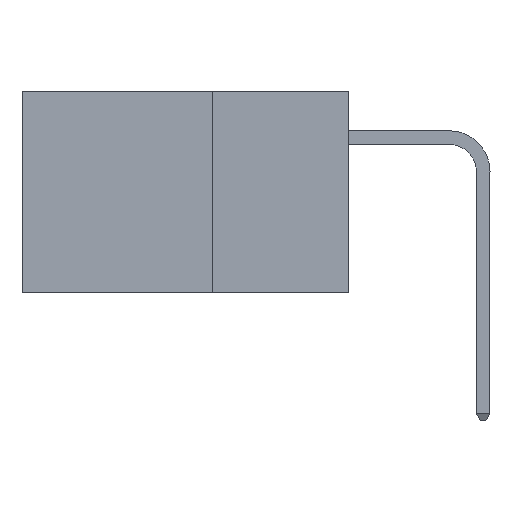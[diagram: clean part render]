
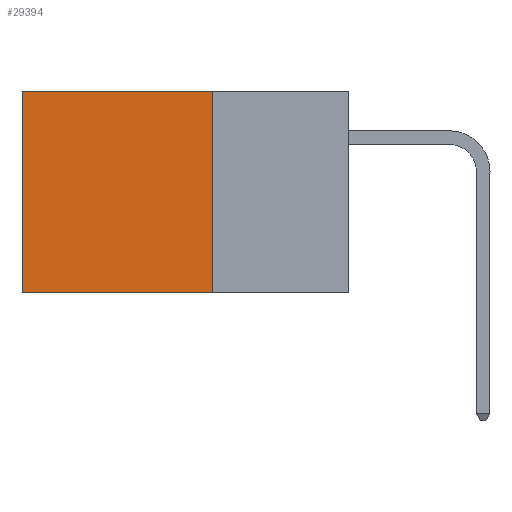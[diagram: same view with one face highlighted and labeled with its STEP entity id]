
A CAD part, left-side view. The second image highlights one B-rep face of the part: STEP entity #29394.
In plain terms, the highlighted planar face has unit normal (-1, 0, 0).
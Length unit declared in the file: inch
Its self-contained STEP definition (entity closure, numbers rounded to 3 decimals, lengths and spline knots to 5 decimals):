
#1461 = DIRECTION ( 'NONE',  ( 0., 0., -1. ) ) ;
#1481 = ORIENTED_EDGE ( 'NONE', *, *, #2013, .T. ) ;
#1617 = VERTEX_POINT ( 'NONE', #10074 ) ;
#2013 = EDGE_CURVE ( 'NONE', #8658, #1617, #14177, .T. ) ;
#5058 = CARTESIAN_POINT ( 'NONE',  ( 0.2875, 0.25, 0. ) ) ;
#5927 = CARTESIAN_POINT ( 'NONE',  ( 0.2875, 0.6, -0.37 ) ) ;
#5929 = VECTOR ( 'NONE', #19101, 39.37008 ) ;
#7107 = CARTESIAN_POINT ( 'NONE',  ( 0.2875, 0.25, -0.37 ) ) ;
#7813 = LINE ( 'NONE', #7107, #5929 ) ;
#8658 = VERTEX_POINT ( 'NONE', #11476 ) ;
#9040 = EDGE_LOOP ( 'NONE', ( #26989, #29808, #34990, #1481 ) ) ;
#10074 = CARTESIAN_POINT ( 'NONE',  ( 0.2875, 0.6, 0. ) ) ;
#11476 = CARTESIAN_POINT ( 'NONE',  ( 0.2875, 0.25, 0. ) ) ;
#12960 = PLANE ( 'NONE',  #15519 ) ;
#14177 = LINE ( 'NONE', #29508, #35835 ) ;
#15425 = VECTOR ( 'NONE', #1461, 39.37008 ) ;
#15519 = AXIS2_PLACEMENT_3D ( 'NONE', #27658, #33579, #15945 ) ;
#15945 = DIRECTION ( 'NONE',  ( 0., 0., -1. ) ) ;
#19101 = DIRECTION ( 'NONE',  ( 0., 1., 0. ) ) ;
#19119 = VERTEX_POINT ( 'NONE', #5927 ) ;
#19145 = FACE_OUTER_BOUND ( 'NONE', #9040, .T. ) ;
#22175 = CARTESIAN_POINT ( 'NONE',  ( 0.2875, 0.6, 0. ) ) ;
#23018 = VECTOR ( 'NONE', #25708, 39.37008 ) ;
#23253 = LINE ( 'NONE', #22175, #15425 ) ;
#23584 = DIRECTION ( 'NONE',  ( 0., 1., 0. ) ) ;
#25708 = DIRECTION ( 'NONE',  ( 0., 0., -1. ) ) ;
#26989 = ORIENTED_EDGE ( 'NONE', *, *, #30607, .T. ) ;
#27197 = EDGE_CURVE ( 'NONE', #8658, #31948, #30874, .T. ) ;
#27658 = CARTESIAN_POINT ( 'NONE',  ( 0.2875, 0.25, 0. ) ) ;
#29394 = ADVANCED_FACE ( 'NONE', ( #19145 ), #12960, .F. ) ;
#29508 = CARTESIAN_POINT ( 'NONE',  ( 0.2875, 0.25, 0. ) ) ;
#29808 = ORIENTED_EDGE ( 'NONE', *, *, #34203, .F. ) ;
#30607 = EDGE_CURVE ( 'NONE', #1617, #19119, #23253, .T. ) ;
#30874 = LINE ( 'NONE', #5058, #23018 ) ;
#31240 = CARTESIAN_POINT ( 'NONE',  ( 0.2875, 0.25, -0.37 ) ) ;
#31948 = VERTEX_POINT ( 'NONE', #31240 ) ;
#33579 = DIRECTION ( 'NONE',  ( 1., 0., 0. ) ) ;
#34203 = EDGE_CURVE ( 'NONE', #31948, #19119, #7813, .T. ) ;
#34990 = ORIENTED_EDGE ( 'NONE', *, *, #27197, .F. ) ;
#35835 = VECTOR ( 'NONE', #23584, 39.37008 ) ;
